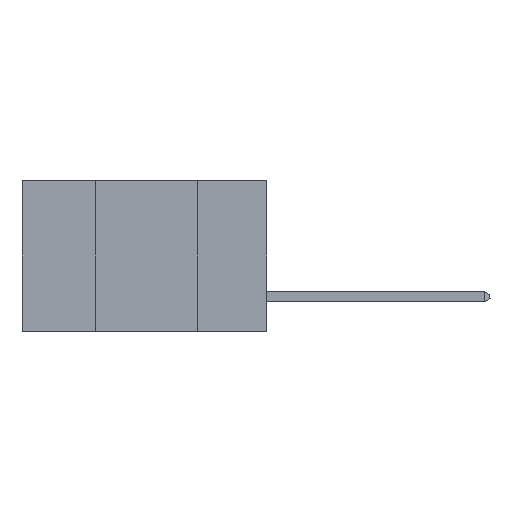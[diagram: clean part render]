
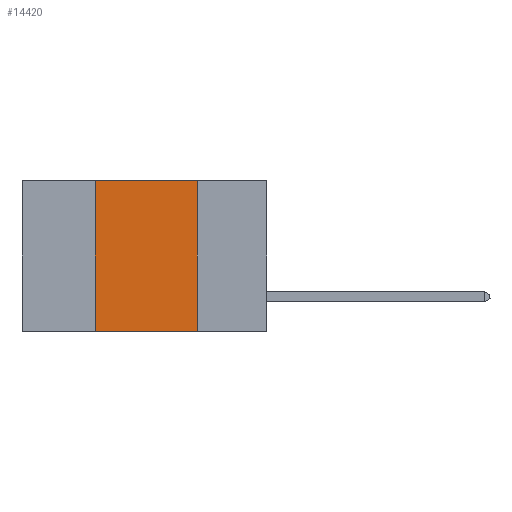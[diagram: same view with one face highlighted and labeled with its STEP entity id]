
A CAD part, left-side view. The second image highlights one B-rep face of the part: STEP entity #14420.
In plain terms, the highlighted planar face has unit normal (-1, 0, 0).
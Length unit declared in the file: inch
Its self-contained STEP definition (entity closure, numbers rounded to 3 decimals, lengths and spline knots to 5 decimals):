
#1248 = PLANE ( 'NONE',  #11660 ) ;
#1280 = LINE ( 'NONE', #13536, #14511 ) ;
#1349 = LINE ( 'NONE', #2564, #18776 ) ;
#1379 = EDGE_CURVE ( 'NONE', #17392, #6491, #12279, .T. ) ;
#1945 = CARTESIAN_POINT ( 'NONE',  ( 0., 0.42, -0.37 ) ) ;
#2368 = LINE ( 'NONE', #19753, #11094 ) ;
#2564 = CARTESIAN_POINT ( 'NONE',  ( 0., 0.17, 0. ) ) ;
#4112 = ORIENTED_EDGE ( 'NONE', *, *, #1379, .T. ) ;
#5298 = VERTEX_POINT ( 'NONE', #15206 ) ;
#5889 = ORIENTED_EDGE ( 'NONE', *, *, #11966, .F. ) ;
#6354 = DIRECTION ( 'NONE',  ( 0., 0., -1. ) ) ;
#6491 = VERTEX_POINT ( 'NONE', #21481 ) ;
#7116 = DIRECTION ( 'NONE',  ( 0., -1., 0. ) ) ;
#7192 = CARTESIAN_POINT ( 'NONE',  ( 0., 0.6, -0.37 ) ) ;
#7734 = EDGE_LOOP ( 'NONE', ( #5889, #16307, #9552, #4112 ) ) ;
#7825 = EDGE_CURVE ( 'NONE', #17392, #13314, #2368, .T. ) ;
#7835 = VECTOR ( 'NONE', #7116, 39.37008 ) ;
#9552 = ORIENTED_EDGE ( 'NONE', *, *, #7825, .F. ) ;
#11094 = VECTOR ( 'NONE', #16217, 39.37008 ) ;
#11660 = AXIS2_PLACEMENT_3D ( 'NONE', #19912, #14640, #6354 ) ;
#11966 = EDGE_CURVE ( 'NONE', #5298, #6491, #1349, .T. ) ;
#12279 = LINE ( 'NONE', #7192, #7835 ) ;
#12994 = FACE_OUTER_BOUND ( 'NONE', #7734, .T. ) ;
#13314 = VERTEX_POINT ( 'NONE', #13481 ) ;
#13481 = CARTESIAN_POINT ( 'NONE',  ( 0., 0.42, 0. ) ) ;
#13536 = CARTESIAN_POINT ( 'NONE',  ( 0., 0.6, 0. ) ) ;
#14420 = ADVANCED_FACE ( 'NONE', ( #12994 ), #1248, .F. ) ;
#14511 = VECTOR ( 'NONE', #20968, 39.37008 ) ;
#14640 = DIRECTION ( 'NONE',  ( 1., 0., 0. ) ) ;
#15206 = CARTESIAN_POINT ( 'NONE',  ( 0., 0.17, 0. ) ) ;
#15231 = EDGE_CURVE ( 'NONE', #13314, #5298, #1280, .T. ) ;
#16083 = DIRECTION ( 'NONE',  ( 0., 0., -1. ) ) ;
#16217 = DIRECTION ( 'NONE',  ( 0., 0., 1. ) ) ;
#16307 = ORIENTED_EDGE ( 'NONE', *, *, #15231, .F. ) ;
#17392 = VERTEX_POINT ( 'NONE', #1945 ) ;
#18776 = VECTOR ( 'NONE', #16083, 39.37008 ) ;
#19753 = CARTESIAN_POINT ( 'NONE',  ( 0., 0.42, 0. ) ) ;
#19912 = CARTESIAN_POINT ( 'NONE',  ( 0., 0.6, 0. ) ) ;
#20968 = DIRECTION ( 'NONE',  ( 0., -1., 0. ) ) ;
#21481 = CARTESIAN_POINT ( 'NONE',  ( 0., 0.17, -0.37 ) ) ;
